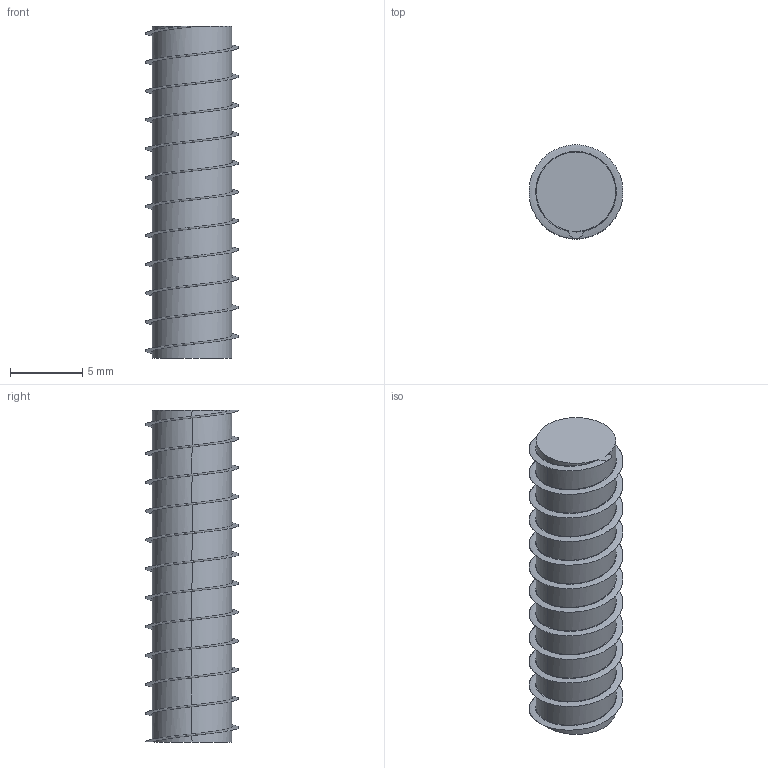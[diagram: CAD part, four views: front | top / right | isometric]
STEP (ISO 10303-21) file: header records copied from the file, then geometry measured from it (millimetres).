
FILE_DESCRIPTION (( 'STEP AP214' ), '1' );
FILE_NAME ('SpringComp^StikM1.STEP', '2013-09-01T22:37:12', ( 'Asher' ), ( '' ), 'SwSTEP 2.0', 'SolidWorks 2013', '' );
FILE_SCHEMA (( 'AUTOMOTIVE_DESIGN' ));
Length unit declared in the file: millimetre
Products named in the file (1): SpringComp^StikM1
Bounding box: 6.5 x 6.5 x 23 mm (x, y, z)
Volume: 555.9 mm3; surface area: 645.2 mm2
Topology: 1 solids, 1 shells, 31 faces, 87 edges, 58 vertices
Faces by surface type: cylinder 26, bspline 3, plane 2
Entity records: 6725 total; most frequent: CARTESIAN_POINT 6037, ORIENTED_EDGE 174, DIRECTION 107, EDGE_CURVE 87, VERTEX_POINT 58, AXIS2_PLACEMENT_3D 41, EDGE_LOOP 31, ADVANCED_FACE 31
